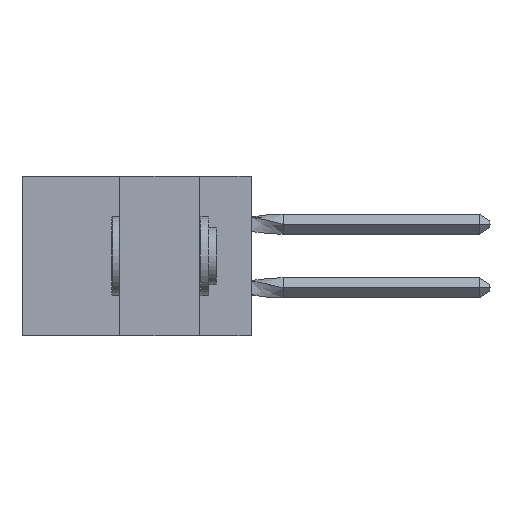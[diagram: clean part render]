
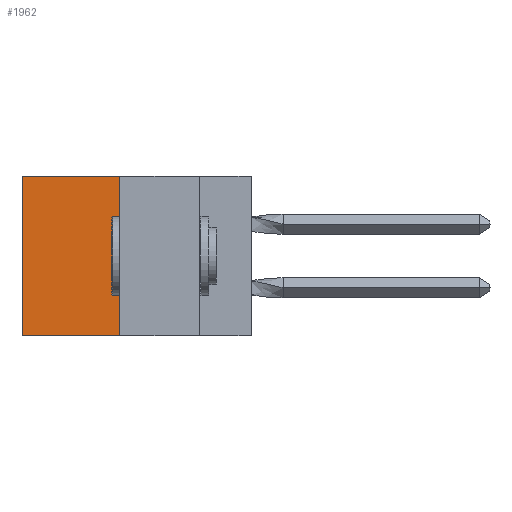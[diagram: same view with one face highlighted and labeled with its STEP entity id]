
A CAD part, left-side view. The second image highlights one B-rep face of the part: STEP entity #1962.
In plain terms, the highlighted planar face has unit normal (-1, 0, 0).
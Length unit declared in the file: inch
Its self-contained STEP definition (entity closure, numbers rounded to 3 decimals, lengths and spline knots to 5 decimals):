
#426 = VERTEX_POINT ( 'NONE', #11636 ) ;
#510 = CARTESIAN_POINT ( 'NONE',  ( 0.305, 0.72, 0. ) ) ;
#1432 = EDGE_CURVE ( 'NONE', #1913, #1674, #13294, .T. ) ;
#1674 = VERTEX_POINT ( 'NONE', #19623 ) ;
#1913 = VERTEX_POINT ( 'NONE', #9573 ) ;
#1962 = ADVANCED_FACE ( 'NONE', ( #19261 ), #11838, .F. ) ;
#2148 = VECTOR ( 'NONE', #20467, 39.37008 ) ;
#2368 = EDGE_CURVE ( 'NONE', #1674, #426, #15687, .T. ) ;
#3595 = EDGE_LOOP ( 'NONE', ( #13335, #9214, #9772, #13946 ) ) ;
#4232 = CARTESIAN_POINT ( 'NONE',  ( 0.305, 0.413, 0. ) ) ;
#4860 = DIRECTION ( 'NONE',  ( 1., 0., 0. ) ) ;
#5723 = LINE ( 'NONE', #17542, #14679 ) ;
#6199 = DIRECTION ( 'NONE',  ( 0., 1., 0. ) ) ;
#6203 = DIRECTION ( 'NONE',  ( 0., 1., 0. ) ) ;
#7794 = VECTOR ( 'NONE', #6203, 39.37008 ) ;
#9214 = ORIENTED_EDGE ( 'NONE', *, *, #2368, .F. ) ;
#9573 = CARTESIAN_POINT ( 'NONE',  ( 0.305, 0.413, 0. ) ) ;
#9772 = ORIENTED_EDGE ( 'NONE', *, *, #1432, .F. ) ;
#10558 = EDGE_CURVE ( 'NONE', #10652, #426, #5723, .T. ) ;
#10617 = CARTESIAN_POINT ( 'NONE',  ( 0.305, 0.413, -0.5 ) ) ;
#10652 = VERTEX_POINT ( 'NONE', #510 ) ;
#11636 = CARTESIAN_POINT ( 'NONE',  ( 0.305, 0.72, -0.5 ) ) ;
#11838 = PLANE ( 'NONE',  #16987 ) ;
#13294 = LINE ( 'NONE', #16961, #2148 ) ;
#13335 = ORIENTED_EDGE ( 'NONE', *, *, #10558, .T. ) ;
#13544 = EDGE_CURVE ( 'NONE', #1913, #10652, #14913, .T. ) ;
#13755 = DIRECTION ( 'NONE',  ( 0., 0., -1. ) ) ;
#13946 = ORIENTED_EDGE ( 'NONE', *, *, #13544, .T. ) ;
#14679 = VECTOR ( 'NONE', #13755, 39.37008 ) ;
#14913 = LINE ( 'NONE', #4232, #15735 ) ;
#15687 = LINE ( 'NONE', #10617, #7794 ) ;
#15735 = VECTOR ( 'NONE', #6199, 39.37008 ) ;
#16961 = CARTESIAN_POINT ( 'NONE',  ( 0.305, 0.413, -0.5 ) ) ;
#16987 = AXIS2_PLACEMENT_3D ( 'NONE', #18934, #4860, #20514 ) ;
#17542 = CARTESIAN_POINT ( 'NONE',  ( 0.305, 0.72, -0.5 ) ) ;
#18934 = CARTESIAN_POINT ( 'NONE',  ( 0.305, 0.413, -0.5 ) ) ;
#19261 = FACE_OUTER_BOUND ( 'NONE', #3595, .T. ) ;
#19623 = CARTESIAN_POINT ( 'NONE',  ( 0.305, 0.413, -0.5 ) ) ;
#20467 = DIRECTION ( 'NONE',  ( 0., 0., -1. ) ) ;
#20514 = DIRECTION ( 'NONE',  ( 0., 0., -1. ) ) ;
